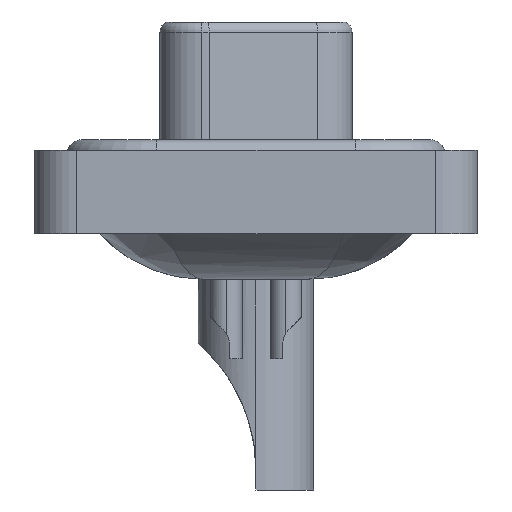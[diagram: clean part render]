
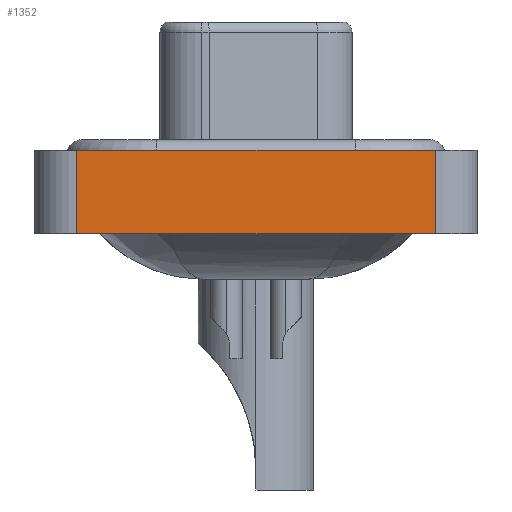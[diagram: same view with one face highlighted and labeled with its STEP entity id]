
A CAD part, left-side view. The second image highlights one B-rep face of the part: STEP entity #1352.
In plain terms, the highlighted planar face has unit normal (-1, 0, 0).
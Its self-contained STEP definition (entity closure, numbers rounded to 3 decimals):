
#342 = EDGE_CURVE ( 'NONE', #5968, #15179, #9056, .T. ) ;
#768 = CARTESIAN_POINT ( 'NONE',  ( -7.25, 8.55, -3.6 ) ) ;
#1352 = ADVANCED_FACE ( 'NONE', ( #16573 ), #15049, .T. ) ;
#1411 = DIRECTION ( 'NONE',  ( 0., 0., 1. ) ) ;
#2829 = CARTESIAN_POINT ( 'NONE',  ( -7.25, -8.55, 0.4 ) ) ;
#4183 = AXIS2_PLACEMENT_3D ( 'NONE', #13771, #5723, #1411 ) ;
#4521 = ORIENTED_EDGE ( 'NONE', *, *, #12852, .T. ) ;
#4525 = CARTESIAN_POINT ( 'NONE',  ( -7.25, -8.55, -3.6 ) ) ;
#4726 = CARTESIAN_POINT ( 'NONE',  ( -7.25, -8.55, -3.6 ) ) ;
#4941 = LINE ( 'NONE', #6204, #14666 ) ;
#5104 = EDGE_CURVE ( 'NONE', #15179, #15598, #4941, .T. ) ;
#5158 = VECTOR ( 'NONE', #12191, 1000. ) ;
#5548 = ORIENTED_EDGE ( 'NONE', *, *, #14373, .T. ) ;
#5723 = DIRECTION ( 'NONE',  ( -1., 0., 0. ) ) ;
#5968 = VERTEX_POINT ( 'NONE', #10314 ) ;
#6111 = DIRECTION ( 'NONE',  ( 0., -1., 0. ) ) ;
#6204 = CARTESIAN_POINT ( 'NONE',  ( -7.25, -8.55, 0.4 ) ) ;
#7210 = LINE ( 'NONE', #4525, #7229 ) ;
#7229 = VECTOR ( 'NONE', #11095, 1000. ) ;
#9056 = LINE ( 'NONE', #768, #17704 ) ;
#9354 = EDGE_LOOP ( 'NONE', ( #4521, #11966, #11551, #5548 ) ) ;
#10314 = CARTESIAN_POINT ( 'NONE',  ( -7.25, 8.55, -3.6 ) ) ;
#11095 = DIRECTION ( 'NONE',  ( 0., -1., 0. ) ) ;
#11208 = CARTESIAN_POINT ( 'NONE',  ( -7.25, 8.55, 0.4 ) ) ;
#11551 = ORIENTED_EDGE ( 'NONE', *, *, #342, .F. ) ;
#11762 = DIRECTION ( 'NONE',  ( 0., 0., 1. ) ) ;
#11966 = ORIENTED_EDGE ( 'NONE', *, *, #5104, .F. ) ;
#12191 = DIRECTION ( 'NONE',  ( 0., 0., 1. ) ) ;
#12280 = CARTESIAN_POINT ( 'NONE',  ( -7.25, -8.55, -3.6 ) ) ;
#12852 = EDGE_CURVE ( 'NONE', #15307, #15598, #14747, .T. ) ;
#13771 = CARTESIAN_POINT ( 'NONE',  ( -7.25, -8.55, -3.6 ) ) ;
#14373 = EDGE_CURVE ( 'NONE', #5968, #15307, #7210, .T. ) ;
#14666 = VECTOR ( 'NONE', #6111, 1000. ) ;
#14747 = LINE ( 'NONE', #12280, #5158 ) ;
#15049 = PLANE ( 'NONE',  #4183 ) ;
#15179 = VERTEX_POINT ( 'NONE', #11208 ) ;
#15307 = VERTEX_POINT ( 'NONE', #4726 ) ;
#15598 = VERTEX_POINT ( 'NONE', #2829 ) ;
#16573 = FACE_OUTER_BOUND ( 'NONE', #9354, .T. ) ;
#17704 = VECTOR ( 'NONE', #11762, 1000. ) ;
